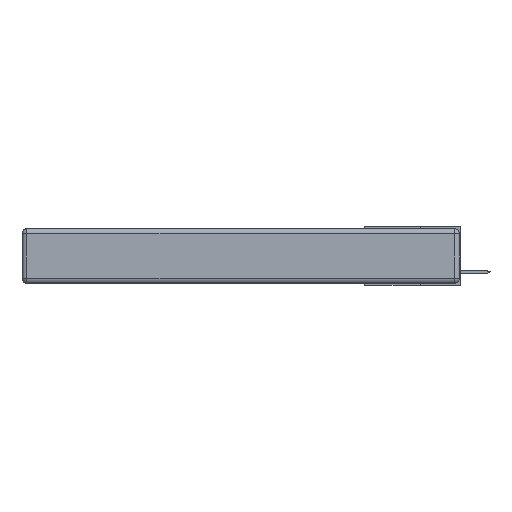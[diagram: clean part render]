
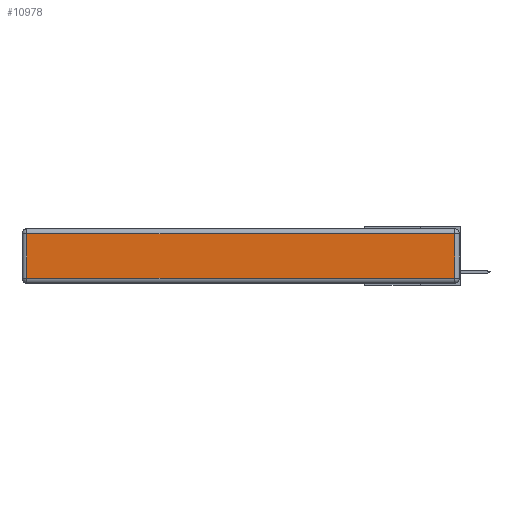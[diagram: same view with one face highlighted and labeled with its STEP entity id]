
A CAD part, left-side view. The second image highlights one B-rep face of the part: STEP entity #10978.
In plain terms, the highlighted planar face has unit normal (-1, 0, 0).
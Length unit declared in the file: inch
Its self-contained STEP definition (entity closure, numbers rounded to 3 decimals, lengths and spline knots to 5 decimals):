
#154 = DIRECTION ( 'NONE',  ( 0., 1., 0. ) ) ;
#695 = EDGE_CURVE ( 'NONE', #18871, #2644, #11458, .T. ) ;
#766 = DIRECTION ( 'NONE',  ( -1., 0., 0. ) ) ;
#891 = CARTESIAN_POINT ( 'NONE',  ( 0., 0., -0.343 ) ) ;
#1649 = ORIENTED_EDGE ( 'NONE', *, *, #9165, .T. ) ;
#2644 = VERTEX_POINT ( 'NONE', #7431 ) ;
#3969 = VECTOR ( 'NONE', #154, 39.37008 ) ;
#3975 = ORIENTED_EDGE ( 'NONE', *, *, #695, .T. ) ;
#5693 = VECTOR ( 'NONE', #20102, 39.37008 ) ;
#6134 = CARTESIAN_POINT ( 'NONE',  ( 0., 0., -0.313 ) ) ;
#6708 = CARTESIAN_POINT ( 'NONE',  ( 0., 2.75, -0.03 ) ) ;
#6737 = CARTESIAN_POINT ( 'NONE',  ( 0., 0.03, -0.313 ) ) ;
#6928 = VECTOR ( 'NONE', #15906, 39.37008 ) ;
#7431 = CARTESIAN_POINT ( 'NONE',  ( 0., 2.72, -0.03 ) ) ;
#7845 = CARTESIAN_POINT ( 'NONE',  ( 0., 0.03, -0.03 ) ) ;
#8712 = FACE_OUTER_BOUND ( 'NONE', #18478, .T. ) ;
#8926 = DIRECTION ( 'NONE',  ( 0., 0., 1. ) ) ;
#9115 = LINE ( 'NONE', #10116, #17038 ) ;
#9165 = EDGE_CURVE ( 'NONE', #11636, #18871, #9115, .T. ) ;
#9598 = VERTEX_POINT ( 'NONE', #20552 ) ;
#10116 = CARTESIAN_POINT ( 'NONE',  ( 0., 0.03, -0.343 ) ) ;
#10722 = LINE ( 'NONE', #6134, #5693 ) ;
#10978 = ADVANCED_FACE ( 'NONE', ( #8712 ), #19932, .T. ) ;
#11458 = LINE ( 'NONE', #6708, #3969 ) ;
#11636 = VERTEX_POINT ( 'NONE', #6737 ) ;
#12395 = LINE ( 'NONE', #12729, #6928 ) ;
#12729 = CARTESIAN_POINT ( 'NONE',  ( 0., 2.72, -0.343 ) ) ;
#15042 = DIRECTION ( 'NONE',  ( 0., 0., 1. ) ) ;
#15906 = DIRECTION ( 'NONE',  ( 0., 0., -1. ) ) ;
#16400 = ORIENTED_EDGE ( 'NONE', *, *, #17407, .T. ) ;
#17038 = VECTOR ( 'NONE', #15042, 39.37008 ) ;
#17407 = EDGE_CURVE ( 'NONE', #9598, #11636, #10722, .T. ) ;
#18478 = EDGE_LOOP ( 'NONE', ( #16400, #1649, #3975, #19133 ) ) ;
#18765 = AXIS2_PLACEMENT_3D ( 'NONE', #891, #766, #8926 ) ;
#18871 = VERTEX_POINT ( 'NONE', #7845 ) ;
#19133 = ORIENTED_EDGE ( 'NONE', *, *, #20139, .T. ) ;
#19932 = PLANE ( 'NONE',  #18765 ) ;
#20102 = DIRECTION ( 'NONE',  ( 0., -1., 0. ) ) ;
#20139 = EDGE_CURVE ( 'NONE', #2644, #9598, #12395, .T. ) ;
#20552 = CARTESIAN_POINT ( 'NONE',  ( 0., 2.72, -0.313 ) ) ;
